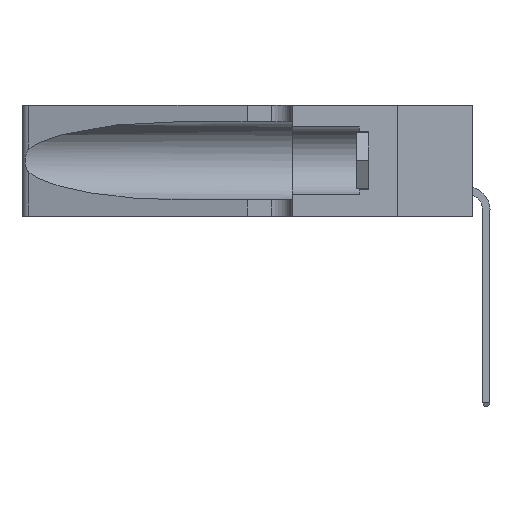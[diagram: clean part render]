
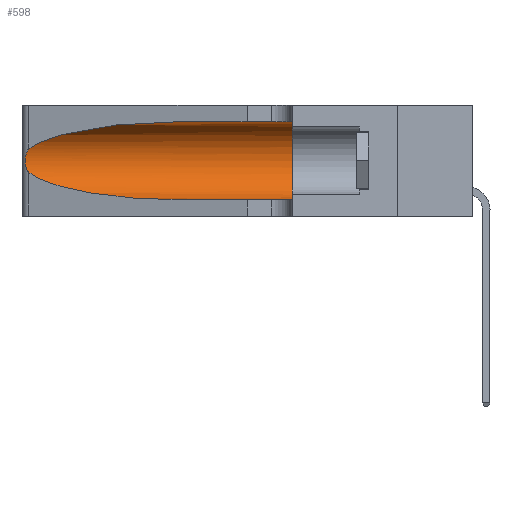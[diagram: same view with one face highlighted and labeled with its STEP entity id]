
A CAD part, left-side view. The second image highlights one B-rep face of the part: STEP entity #598.
In plain terms, the highlighted cylindrical face has radius 3.308 mm (diameter 6.617 mm), a partial arc.
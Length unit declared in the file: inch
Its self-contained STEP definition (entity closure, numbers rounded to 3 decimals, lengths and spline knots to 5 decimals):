
#598 = ADVANCED_FACE ( 'NONE', ( #13417 ), #15163, .F. ) ;
#798 =( BOUNDED_CURVE ( )  B_SPLINE_CURVE ( 3, ( #866, #15054, #6898, #15170 ),
 .UNSPECIFIED., .F., .T. ) 
 B_SPLINE_CURVE_WITH_KNOTS ( ( 4, 4 ),
 ( 3.44316, 4.71239 ),
 .UNSPECIFIED. ) 
 CURVE ( )  GEOMETRIC_REPRESENTATION_ITEM ( )  RATIONAL_B_SPLINE_CURVE ( ( 1., 0.87, 0.87, 1. ) ) 
 REPRESENTATION_ITEM ( '' )  );
#866 = CARTESIAN_POINT ( 'NONE',  ( 0.25487, 1.22718, 0.14631 ) ) ;
#1959 = CARTESIAN_POINT ( 'NONE',  ( 0.26017, 1.23833, 0.17102 ) ) ;
#2453 = CARTESIAN_POINT ( 'NONE',  ( 0.1305, 0.35, 0.185 ) ) ;
#2642 = CARTESIAN_POINT ( 'NONE',  ( 0.25639, 1.23184, 0.21858 ) ) ;
#2693 = CARTESIAN_POINT ( 'NONE',  ( 0.1305, 0.72297, 0.31525 ) ) ;
#3081 = CARTESIAN_POINT ( 'NONE',  ( 0.25555, 1.22994, 0.2215 ) ) ;
#3192 = CARTESIAN_POINT ( 'NONE',  ( 0.25555, 1.22993, 0.14849 ) ) ;
#3338 = EDGE_CURVE ( 'NONE', #30720, #20706, #18509, .T. ) ;
#4010 = CARTESIAN_POINT ( 'NONE',  ( 0.25787, 1.23484, 0.2124 ) ) ;
#4220 = ORIENTED_EDGE ( 'NONE', *, *, #18812, .T. ) ;
#4293 = CARTESIAN_POINT ( 'NONE',  ( 0.1305, 0.72297, 0.05475 ) ) ;
#5344 = ORIENTED_EDGE ( 'NONE', *, *, #34805, .T. ) ;
#6841 = VECTOR ( 'NONE', #25025, 39.37008 ) ;
#6898 = CARTESIAN_POINT ( 'NONE',  ( 0.18966, 0.96281, 0.05475 ) ) ;
#7214 = CARTESIAN_POINT ( 'NONE',  ( 0.25487, 1.22718, 0.22369 ) ) ;
#7327 = CARTESIAN_POINT ( 'NONE',  ( 0.25854, 1.2359, 0.20912 ) ) ;
#7424 = CARTESIAN_POINT ( 'NONE',  ( 0.1305, 0.35, 0.05475 ) ) ;
#7428 = DIRECTION ( 'NONE',  ( 0., -1., 0. ) ) ;
#7603 = CARTESIAN_POINT ( 'NONE',  ( 0.25789, 1.23486, 0.15765 ) ) ;
#8091 = CARTESIAN_POINT ( 'NONE',  ( 0.2373, 1.15595, 0.28018 ) ) ;
#10768 = EDGE_CURVE ( 'NONE', #12038, #13204, #18883, .T. ) ;
#10930 = VERTEX_POINT ( 'NONE', #29678 ) ;
#12038 = VERTEX_POINT ( 'NONE', #26908 ) ;
#13204 = VERTEX_POINT ( 'NONE', #7214 ) ;
#13417 = FACE_OUTER_BOUND ( 'NONE', #26164, .T. ) ;
#14397 = AXIS2_PLACEMENT_3D ( 'NONE', #2453, #19183, #33020 ) ;
#14425 = EDGE_CURVE ( 'NONE', #13204, #10930, #30742, .T. ) ;
#14790 = CARTESIAN_POINT ( 'NONE',  ( 0.26075, 1.23896, 0.178 ) ) ;
#15038 = CARTESIAN_POINT ( 'NONE',  ( 0.25487, 1.22718, 0.14631 ) ) ;
#15054 = CARTESIAN_POINT ( 'NONE',  ( 0.2373, 1.15595, 0.08982 ) ) ;
#15163 = CYLINDRICAL_SURFACE ( 'NONE', #22089, 0.13025 ) ;
#15170 = CARTESIAN_POINT ( 'NONE',  ( 0.1305, 0.72297, 0.05475 ) ) ;
#15706 = CARTESIAN_POINT ( 'NONE',  ( 0.1305, 1.61858, 0.185 ) ) ;
#15800 = LINE ( 'NONE', #16033, #31140 ) ;
#16033 = CARTESIAN_POINT ( 'NONE',  ( 0.1305, 1.61858, 0.05475 ) ) ;
#18081 = ORIENTED_EDGE ( 'NONE', *, *, #14425, .T. ) ;
#18509 = CIRCLE ( 'NONE', #14397, 0.13025 ) ;
#18555 = ORIENTED_EDGE ( 'NONE', *, *, #28535, .F. ) ;
#18812 = EDGE_CURVE ( 'NONE', #31403, #20706, #15800, .T. ) ;
#18883 =( BOUNDED_CURVE ( )  B_SPLINE_CURVE ( 3, ( #2693, #33274, #8091, #28088 ),
 .UNSPECIFIED., .F., .T. ) 
 B_SPLINE_CURVE_WITH_KNOTS ( ( 4, 4 ),
 ( 1.5708, 2.84003 ),
 .UNSPECIFIED. ) 
 CURVE ( )  GEOMETRIC_REPRESENTATION_ITEM ( )  RATIONAL_B_SPLINE_CURVE ( ( 1., 0.87, 0.87, 1. ) ) 
 REPRESENTATION_ITEM ( '' )  );
#19183 = DIRECTION ( 'NONE',  ( 0., 1., 0. ) ) ;
#19966 = ORIENTED_EDGE ( 'NONE', *, *, #3338, .F. ) ;
#20706 = VERTEX_POINT ( 'NONE', #7424 ) ;
#22089 = AXIS2_PLACEMENT_3D ( 'NONE', #15706, #7428, #35284 ) ;
#25025 = DIRECTION ( 'NONE',  ( 0., -1., 0. ) ) ;
#25370 = CARTESIAN_POINT ( 'NONE',  ( 0.1305, 1.61858, 0.31525 ) ) ;
#25452 = CARTESIAN_POINT ( 'NONE',  ( 0.25487, 1.22718, 0.22369 ) ) ;
#26164 = EDGE_LOOP ( 'NONE', ( #34651, #18081, #5344, #4220, #19966, #18555 ) ) ;
#26633 = LINE ( 'NONE', #25370, #6841 ) ;
#26908 = CARTESIAN_POINT ( 'NONE',  ( 0.1305, 0.72297, 0.31525 ) ) ;
#28088 = CARTESIAN_POINT ( 'NONE',  ( 0.25487, 1.22718, 0.22369 ) ) ;
#28535 = EDGE_CURVE ( 'NONE', #12038, #30720, #26633, .T. ) ;
#28892 = CARTESIAN_POINT ( 'NONE',  ( 0.1305, 0.35, 0.31525 ) ) ;
#29035 = CARTESIAN_POINT ( 'NONE',  ( 0.26075, 1.23896, 0.19203 ) ) ;
#29678 = CARTESIAN_POINT ( 'NONE',  ( 0.25487, 1.22718, 0.14631 ) ) ;
#30720 = VERTEX_POINT ( 'NONE', #28892 ) ;
#30742 = B_SPLINE_CURVE_WITH_KNOTS ( 'NONE', 3,
 ( #25452, #3081, #2642, #4010, #7327, #33114, #29035, #14790, #1959, #35051, #7603, #36069, #3192, #15038 ),
 .UNSPECIFIED., .F., .F.,
 ( 4, 2, 2, 2, 2, 2, 4 ),
 ( 0., 0.00027, 0.00053, 0.00107, 0.0016, 0.00187, 0.00214 ),
 .UNSPECIFIED. ) ;
#31140 = VECTOR ( 'NONE', #33060, 39.37008 ) ;
#31403 = VERTEX_POINT ( 'NONE', #4293 ) ;
#33020 = DIRECTION ( 'NONE',  ( 0., 0., 1. ) ) ;
#33060 = DIRECTION ( 'NONE',  ( 0., -1., 0. ) ) ;
#33114 = CARTESIAN_POINT ( 'NONE',  ( 0.26018, 1.23835, 0.19895 ) ) ;
#33274 = CARTESIAN_POINT ( 'NONE',  ( 0.18966, 0.96281, 0.31525 ) ) ;
#34651 = ORIENTED_EDGE ( 'NONE', *, *, #10768, .T. ) ;
#34805 = EDGE_CURVE ( 'NONE', #10930, #31403, #798, .T. ) ;
#35051 = CARTESIAN_POINT ( 'NONE',  ( 0.25856, 1.23593, 0.16098 ) ) ;
#35284 = DIRECTION ( 'NONE',  ( 0., 0., -1. ) ) ;
#36069 = CARTESIAN_POINT ( 'NONE',  ( 0.25639, 1.23186, 0.15144 ) ) ;
